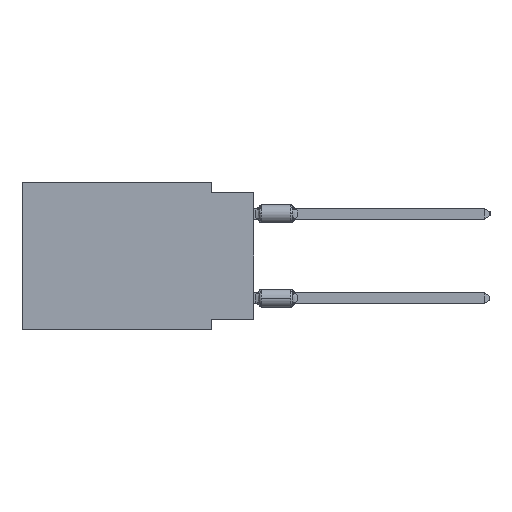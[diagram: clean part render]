
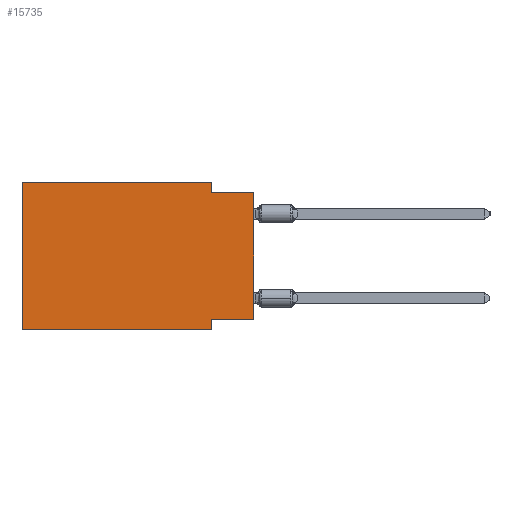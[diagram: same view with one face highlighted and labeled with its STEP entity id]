
A CAD part, left-side view. The second image highlights one B-rep face of the part: STEP entity #15735.
In plain terms, the highlighted planar face has unit normal (-1, 0, 0).
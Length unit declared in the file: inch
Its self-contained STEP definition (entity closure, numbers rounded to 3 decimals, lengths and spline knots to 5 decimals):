
#596 = VECTOR ( 'NONE', #15719, 39.37008 ) ;
#622 = AXIS2_PLACEMENT_3D ( 'NONE', #9861, #6315, #9662 ) ;
#1178 = LINE ( 'NONE', #13746, #21703 ) ;
#1666 = VECTOR ( 'NONE', #12048, 39.37008 ) ;
#2300 = EDGE_CURVE ( 'NONE', #16166, #18291, #31276, .T. ) ;
#3088 = LINE ( 'NONE', #3692, #5416 ) ;
#3308 = VECTOR ( 'NONE', #38094, 39.37008 ) ;
#3385 = FACE_OUTER_BOUND ( 'NONE', #36854, .T. ) ;
#3405 = VERTEX_POINT ( 'NONE', #26721 ) ;
#3692 = CARTESIAN_POINT ( 'NONE',  ( 0., 0.1, -0.35 ) ) ;
#4114 = DIRECTION ( 'NONE',  ( 0., 0., 1. ) ) ;
#5125 = CARTESIAN_POINT ( 'NONE',  ( 0., 0., -0.025 ) ) ;
#5416 = VECTOR ( 'NONE', #38585, 39.37008 ) ;
#5989 = ORIENTED_EDGE ( 'NONE', *, *, #32519, .F. ) ;
#6260 = EDGE_CURVE ( 'NONE', #3405, #32041, #1178, .T. ) ;
#6271 = CARTESIAN_POINT ( 'NONE',  ( 0., 0.1, 0. ) ) ;
#6315 = DIRECTION ( 'NONE',  ( 1., 0., 0. ) ) ;
#6672 = LINE ( 'NONE', #35496, #596 ) ;
#7638 = VECTOR ( 'NONE', #40755, 39.37008 ) ;
#9662 = DIRECTION ( 'NONE',  ( 0., 0., -1. ) ) ;
#9746 = VERTEX_POINT ( 'NONE', #14678 ) ;
#9861 = CARTESIAN_POINT ( 'NONE',  ( 0., 0.55, 0. ) ) ;
#10995 = LINE ( 'NONE', #5125, #20577 ) ;
#12048 = DIRECTION ( 'NONE',  ( 0., -1., 0. ) ) ;
#13124 = ORIENTED_EDGE ( 'NONE', *, *, #19856, .T. ) ;
#13672 = ORIENTED_EDGE ( 'NONE', *, *, #36383, .F. ) ;
#13746 = CARTESIAN_POINT ( 'NONE',  ( 0., 0.55, 0. ) ) ;
#14678 = CARTESIAN_POINT ( 'NONE',  ( 0., 0.1, -0.35 ) ) ;
#15010 = CARTESIAN_POINT ( 'NONE',  ( 0., 0.1, 0. ) ) ;
#15072 = VERTEX_POINT ( 'NONE', #35895 ) ;
#15301 = LINE ( 'NONE', #20940, #7638 ) ;
#15304 = CARTESIAN_POINT ( 'NONE',  ( 0., 0., -0.325 ) ) ;
#15719 = DIRECTION ( 'NONE',  ( 0., -1., 0. ) ) ;
#15735 = ADVANCED_FACE ( 'NONE', ( #3385 ), #38086, .F. ) ;
#16119 = EDGE_CURVE ( 'NONE', #32041, #16166, #6672, .T. ) ;
#16166 = VERTEX_POINT ( 'NONE', #6271 ) ;
#17098 = CARTESIAN_POINT ( 'NONE',  ( 0., 0.1, -0.025 ) ) ;
#17568 = EDGE_CURVE ( 'NONE', #38019, #15072, #15301, .T. ) ;
#18291 = VERTEX_POINT ( 'NONE', #17098 ) ;
#18545 = LINE ( 'NONE', #34403, #1666 ) ;
#19856 = EDGE_CURVE ( 'NONE', #3405, #9746, #18545, .T. ) ;
#20515 = ORIENTED_EDGE ( 'NONE', *, *, #2300, .F. ) ;
#20577 = VECTOR ( 'NONE', #40022, 39.37008 ) ;
#20940 = CARTESIAN_POINT ( 'NONE',  ( 0., 0., 0. ) ) ;
#21703 = VECTOR ( 'NONE', #4114, 39.37008 ) ;
#22250 = CARTESIAN_POINT ( 'NONE',  ( 0., 0., -0.325 ) ) ;
#22413 = ORIENTED_EDGE ( 'NONE', *, *, #17568, .T. ) ;
#22651 = LINE ( 'NONE', #22250, #3308 ) ;
#23408 = CARTESIAN_POINT ( 'NONE',  ( 0., 0.55, 0. ) ) ;
#26520 = ORIENTED_EDGE ( 'NONE', *, *, #6260, .F. ) ;
#26721 = CARTESIAN_POINT ( 'NONE',  ( 0., 0.55, -0.35 ) ) ;
#27678 = VECTOR ( 'NONE', #40465, 39.37008 ) ;
#27959 = VERTEX_POINT ( 'NONE', #33439 ) ;
#28645 = EDGE_CURVE ( 'NONE', #27959, #9746, #3088, .T. ) ;
#30608 = ORIENTED_EDGE ( 'NONE', *, *, #16119, .F. ) ;
#31276 = LINE ( 'NONE', #15010, #27678 ) ;
#31763 = ORIENTED_EDGE ( 'NONE', *, *, #28645, .F. ) ;
#32041 = VERTEX_POINT ( 'NONE', #23408 ) ;
#32519 = EDGE_CURVE ( 'NONE', #18291, #15072, #10995, .T. ) ;
#33439 = CARTESIAN_POINT ( 'NONE',  ( 0., 0.1, -0.325 ) ) ;
#34403 = CARTESIAN_POINT ( 'NONE',  ( 0., 0.55, -0.35 ) ) ;
#35496 = CARTESIAN_POINT ( 'NONE',  ( 0., 0.55, 0. ) ) ;
#35895 = CARTESIAN_POINT ( 'NONE',  ( 0., 0., -0.025 ) ) ;
#36383 = EDGE_CURVE ( 'NONE', #38019, #27959, #22651, .T. ) ;
#36854 = EDGE_LOOP ( 'NONE', ( #22413, #5989, #20515, #30608, #26520, #13124, #31763, #13672 ) ) ;
#38019 = VERTEX_POINT ( 'NONE', #15304 ) ;
#38086 = PLANE ( 'NONE',  #622 ) ;
#38094 = DIRECTION ( 'NONE',  ( 0., 1., 0. ) ) ;
#38585 = DIRECTION ( 'NONE',  ( 0., 0., -1. ) ) ;
#40022 = DIRECTION ( 'NONE',  ( 0., -1., 0. ) ) ;
#40465 = DIRECTION ( 'NONE',  ( 0., 0., -1. ) ) ;
#40755 = DIRECTION ( 'NONE',  ( 0., 0., 1. ) ) ;
